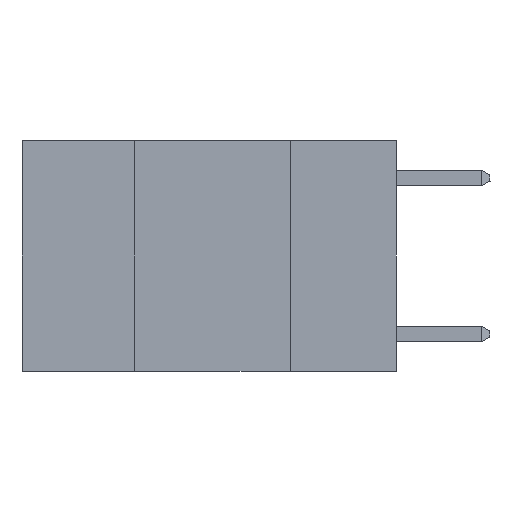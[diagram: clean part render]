
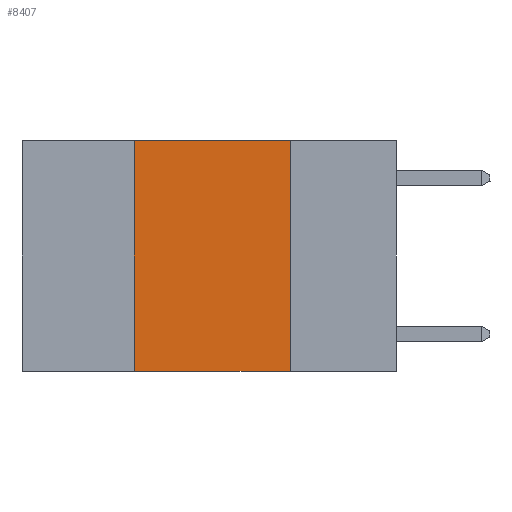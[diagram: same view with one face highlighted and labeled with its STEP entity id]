
A CAD part, left-side view. The second image highlights one B-rep face of the part: STEP entity #8407.
In plain terms, the highlighted planar face has unit normal (-1, 0, 0).
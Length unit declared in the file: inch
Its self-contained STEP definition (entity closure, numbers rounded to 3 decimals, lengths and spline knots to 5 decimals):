
#350 = DIRECTION ( 'NONE',  ( 0., 0., -1. ) ) ;
#483 = VECTOR ( 'NONE', #7105, 39.37008 ) ;
#867 = CARTESIAN_POINT ( 'NONE',  ( 0., 0.17, 0. ) ) ;
#2984 = EDGE_CURVE ( 'NONE', #23575, #10611, #10984, .T. ) ;
#3089 = EDGE_LOOP ( 'NONE', ( #17911, #18160, #18190, #18265 ) ) ;
#4162 = VECTOR ( 'NONE', #8615, 39.37008 ) ;
#4293 = AXIS2_PLACEMENT_3D ( 'NONE', #22577, #11660, #350 ) ;
#4993 = LINE ( 'NONE', #18113, #483 ) ;
#5506 = EDGE_CURVE ( 'NONE', #10611, #9925, #13192, .T. ) ;
#6981 = DIRECTION ( 'NONE',  ( 0., -1., 0. ) ) ;
#7105 = DIRECTION ( 'NONE',  ( 0., -1., 0. ) ) ;
#8407 = ADVANCED_FACE ( 'NONE', ( #18801 ), #13413, .F. ) ;
#8615 = DIRECTION ( 'NONE',  ( 0., 0., -1. ) ) ;
#8618 = VERTEX_POINT ( 'NONE', #21342 ) ;
#8992 = DIRECTION ( 'NONE',  ( 0., 0., 1. ) ) ;
#9925 = VERTEX_POINT ( 'NONE', #867 ) ;
#9955 = EDGE_CURVE ( 'NONE', #9925, #8618, #23137, .T. ) ;
#10611 = VERTEX_POINT ( 'NONE', #15288 ) ;
#10633 = CARTESIAN_POINT ( 'NONE',  ( 0., 0.42, -0.37 ) ) ;
#10984 = LINE ( 'NONE', #19984, #15858 ) ;
#11660 = DIRECTION ( 'NONE',  ( 1., 0., 0. ) ) ;
#12055 = VECTOR ( 'NONE', #6981, 39.37008 ) ;
#13192 = LINE ( 'NONE', #16142, #12055 ) ;
#13413 = PLANE ( 'NONE',  #4293 ) ;
#15288 = CARTESIAN_POINT ( 'NONE',  ( 0., 0.42, 0. ) ) ;
#15858 = VECTOR ( 'NONE', #8992, 39.37008 ) ;
#16142 = CARTESIAN_POINT ( 'NONE',  ( 0., 0.6, 0. ) ) ;
#17271 = EDGE_CURVE ( 'NONE', #23575, #8618, #4993, .T. ) ;
#17911 = ORIENTED_EDGE ( 'NONE', *, *, #9955, .F. ) ;
#18113 = CARTESIAN_POINT ( 'NONE',  ( 0., 0.6, -0.37 ) ) ;
#18160 = ORIENTED_EDGE ( 'NONE', *, *, #5506, .F. ) ;
#18190 = ORIENTED_EDGE ( 'NONE', *, *, #2984, .F. ) ;
#18265 = ORIENTED_EDGE ( 'NONE', *, *, #17271, .T. ) ;
#18801 = FACE_OUTER_BOUND ( 'NONE', #3089, .T. ) ;
#19984 = CARTESIAN_POINT ( 'NONE',  ( 0., 0.42, 0. ) ) ;
#21342 = CARTESIAN_POINT ( 'NONE',  ( 0., 0.17, -0.37 ) ) ;
#21362 = CARTESIAN_POINT ( 'NONE',  ( 0., 0.17, 0. ) ) ;
#22577 = CARTESIAN_POINT ( 'NONE',  ( 0., 0.6, 0. ) ) ;
#23137 = LINE ( 'NONE', #21362, #4162 ) ;
#23575 = VERTEX_POINT ( 'NONE', #10633 ) ;
